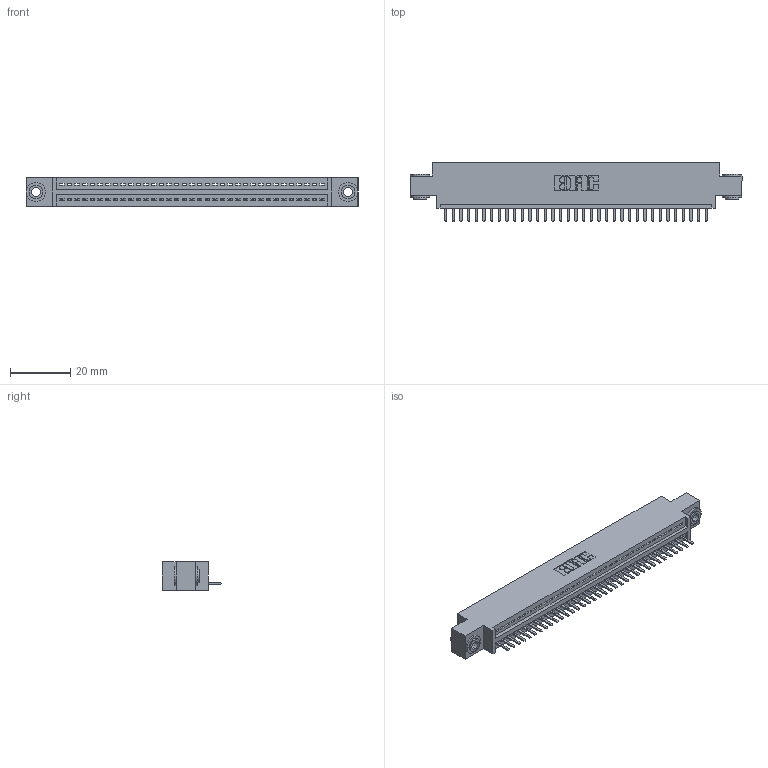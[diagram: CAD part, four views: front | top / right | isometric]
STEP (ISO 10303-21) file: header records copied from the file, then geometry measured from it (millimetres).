
FILE_DESCRIPTION (( 'STEP AP203' ), '1' );
FILE_NAME ('345-035-520-603.STEP', '2018-08-29T05:42:37', ( '' ), ( '' ), 'SwSTEP 2.0', 'SolidWorks 2016', '' );
FILE_SCHEMA (( 'CONFIG_CONTROL_DESIGN' ));
Length unit declared in the file: inch
Products named in the file (4): 345 Part_0.170 Offset - 0.156 Dia-TH; 345-292-001_345-293-120; 345-250-002_345-250-002-102; 345-035-520-603
Assembly tree (38 placements, depth 2):
  345-035-520-603
    345 Part_0.170 Offset - 0.156 Dia-TH
    345-292-001_345-293-120  x35
    345-250-002_345-250-002-102  x2
Bounding box: 110.11 x 19.68 x 9.4 mm (x, y, z)
Volume: 10206.3 mm3; surface area: 13479.7 mm2
Topology: 38 solids, 38 shells, 2338 faces, 6869 edges, 4482 vertices
Faces by surface type: plane 1564, cylinder 766, cone 8
Entity records: 28180 total; most frequent: CARTESIAN_POINT 4872, ORIENTED_EDGE 4822, DIRECTION 4283, EDGE_CURVE 2411, VECTOR 2111, LINE 2111, VERTEX_POINT 1602, AXIS2_PLACEMENT_3D 1086
